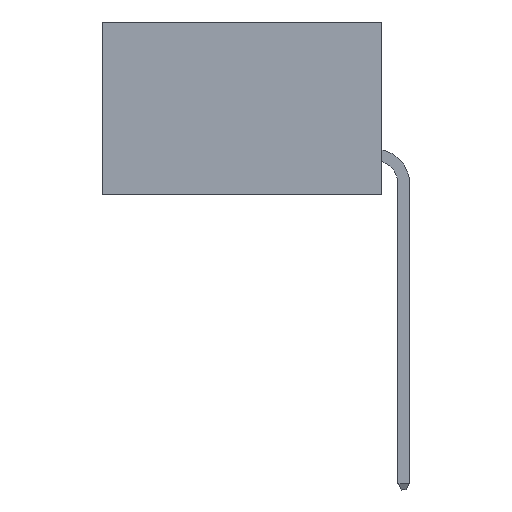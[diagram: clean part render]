
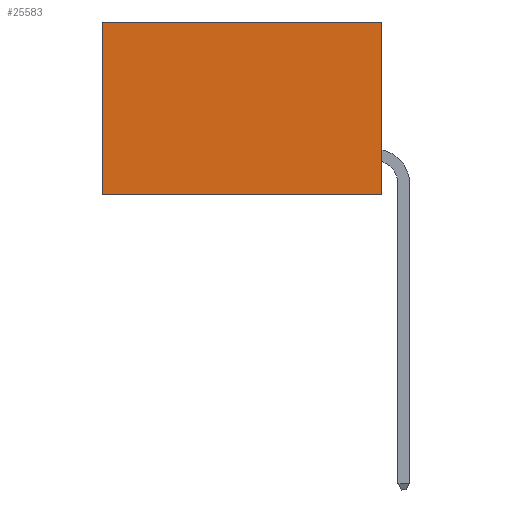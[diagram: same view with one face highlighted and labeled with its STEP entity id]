
A CAD part, left-side view. The second image highlights one B-rep face of the part: STEP entity #25583.
In plain terms, the highlighted planar face has unit normal (-1, 0, 0).
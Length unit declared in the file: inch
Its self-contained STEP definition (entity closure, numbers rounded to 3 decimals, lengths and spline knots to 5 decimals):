
#947 = ORIENTED_EDGE ( 'NONE', *, *, #3111, .F. ) ;
#1481 = EDGE_LOOP ( 'NONE', ( #21189, #947, #10973, #4720 ) ) ;
#1737 = CARTESIAN_POINT ( 'NONE',  ( 0.2875, 0., 0. ) ) ;
#2818 = VECTOR ( 'NONE', #25472, 39.37008 ) ;
#3111 = EDGE_CURVE ( 'NONE', #23258, #30606, #11500, .T. ) ;
#4320 = CARTESIAN_POINT ( 'NONE',  ( 0.2875, 0., 0. ) ) ;
#4720 = ORIENTED_EDGE ( 'NONE', *, *, #28018, .T. ) ;
#5045 = FACE_OUTER_BOUND ( 'NONE', #1481, .T. ) ;
#5196 = CARTESIAN_POINT ( 'NONE',  ( 0.2875, 0., 0. ) ) ;
#5261 = LINE ( 'NONE', #1737, #17369 ) ;
#9207 = DIRECTION ( 'NONE',  ( 0., 0., -1. ) ) ;
#9850 = CARTESIAN_POINT ( 'NONE',  ( 0.2875, 0., 0. ) ) ;
#9941 = CARTESIAN_POINT ( 'NONE',  ( 0.2875, 0., -0.37 ) ) ;
#10538 = VECTOR ( 'NONE', #21957, 39.37008 ) ;
#10747 = VECTOR ( 'NONE', #24767, 39.37008 ) ;
#10973 = ORIENTED_EDGE ( 'NONE', *, *, #19786, .F. ) ;
#11500 = LINE ( 'NONE', #9941, #10747 ) ;
#12321 = DIRECTION ( 'NONE',  ( 0., 0., -1. ) ) ;
#14095 = CARTESIAN_POINT ( 'NONE',  ( 0.2875, 0.6, -0.37 ) ) ;
#15427 = LINE ( 'NONE', #5196, #10538 ) ;
#15603 = CARTESIAN_POINT ( 'NONE',  ( 0.2875, 0.6, 0. ) ) ;
#17369 = VECTOR ( 'NONE', #9207, 39.37008 ) ;
#18201 = CARTESIAN_POINT ( 'NONE',  ( 0.2875, 0.6, 0. ) ) ;
#18243 = AXIS2_PLACEMENT_3D ( 'NONE', #9850, #26678, #12321 ) ;
#19786 = EDGE_CURVE ( 'NONE', #27834, #23258, #5261, .T. ) ;
#21189 = ORIENTED_EDGE ( 'NONE', *, *, #21753, .T. ) ;
#21753 = EDGE_CURVE ( 'NONE', #26440, #30606, #22152, .T. ) ;
#21794 = PLANE ( 'NONE',  #18243 ) ;
#21957 = DIRECTION ( 'NONE',  ( 0., 1., 0. ) ) ;
#22152 = LINE ( 'NONE', #18201, #2818 ) ;
#23258 = VERTEX_POINT ( 'NONE', #25720 ) ;
#24767 = DIRECTION ( 'NONE',  ( 0., 1., 0. ) ) ;
#25472 = DIRECTION ( 'NONE',  ( 0., 0., -1. ) ) ;
#25583 = ADVANCED_FACE ( 'NONE', ( #5045 ), #21794, .F. ) ;
#25720 = CARTESIAN_POINT ( 'NONE',  ( 0.2875, 0., -0.37 ) ) ;
#26440 = VERTEX_POINT ( 'NONE', #15603 ) ;
#26678 = DIRECTION ( 'NONE',  ( 1., 0., 0. ) ) ;
#27834 = VERTEX_POINT ( 'NONE', #4320 ) ;
#28018 = EDGE_CURVE ( 'NONE', #27834, #26440, #15427, .T. ) ;
#30606 = VERTEX_POINT ( 'NONE', #14095 ) ;
